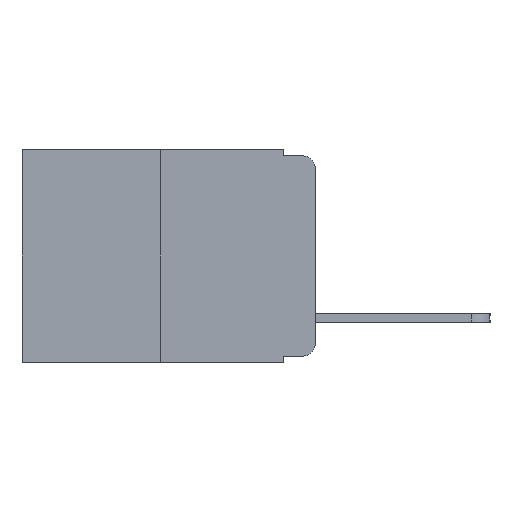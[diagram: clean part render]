
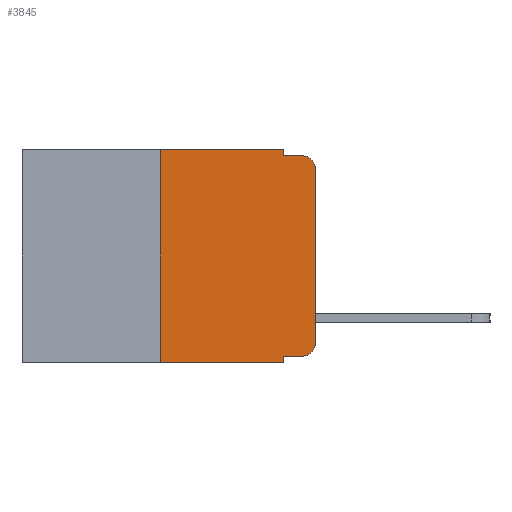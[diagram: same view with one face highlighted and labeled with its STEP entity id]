
A CAD part, left-side view. The second image highlights one B-rep face of the part: STEP entity #3845.
In plain terms, the highlighted planar face has unit normal (-1, 0, 0).
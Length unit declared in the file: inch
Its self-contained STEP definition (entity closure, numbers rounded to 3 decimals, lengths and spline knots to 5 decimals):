
#134 = LINE ( 'NONE', #8582, #2437 ) ;
#140 = DIRECTION ( 'NONE',  ( 0., 0., -1. ) ) ;
#156 = AXIS2_PLACEMENT_3D ( 'NONE', #11019, #10996, #140 ) ;
#361 = ORIENTED_EDGE ( 'NONE', *, *, #5059, .F. ) ;
#370 = EDGE_CURVE ( 'NONE', #8554, #5490, #8906, .T. ) ;
#507 = VECTOR ( 'NONE', #10525, 39.37008 ) ;
#879 = EDGE_CURVE ( 'NONE', #2449, #7760, #5475, .T. ) ;
#1166 = ORIENTED_EDGE ( 'NONE', *, *, #9268, .T. ) ;
#1255 = VERTEX_POINT ( 'NONE', #6982 ) ;
#1303 = CARTESIAN_POINT ( 'NONE',  ( 0., 0.051, -0.333 ) ) ;
#1473 = ORIENTED_EDGE ( 'NONE', *, *, #1939, .T. ) ;
#1610 = EDGE_CURVE ( 'NONE', #2449, #7547, #134, .T. ) ;
#1615 = ORIENTED_EDGE ( 'NONE', *, *, #8835, .F. ) ;
#1650 = CARTESIAN_POINT ( 'NONE',  ( 0., 0., 0. ) ) ;
#1878 = EDGE_CURVE ( 'NONE', #9901, #1255, #3723, .T. ) ;
#1939 = EDGE_CURVE ( 'NONE', #5402, #5490, #5911, .T. ) ;
#1946 = LINE ( 'NONE', #7450, #8960 ) ;
#2437 = VECTOR ( 'NONE', #9664, 39.37008 ) ;
#2449 = VERTEX_POINT ( 'NONE', #6553 ) ;
#2510 = CARTESIAN_POINT ( 'NONE',  ( 0., 0.02, -0.313 ) ) ;
#3001 = AXIS2_PLACEMENT_3D ( 'NONE', #9439, #4034, #8650 ) ;
#3351 = ORIENTED_EDGE ( 'NONE', *, *, #1610, .T. ) ;
#3541 = VECTOR ( 'NONE', #6792, 39.37008 ) ;
#3632 = EDGE_CURVE ( 'NONE', #7420, #9901, #7982, .T. ) ;
#3723 = CIRCLE ( 'NONE', #7213, 0.02 ) ;
#3845 = ADVANCED_FACE ( 'NONE', ( #10465 ), #3967, .F. ) ;
#3888 = DIRECTION ( 'NONE',  ( 0., -1., 0. ) ) ;
#3967 = PLANE ( 'NONE',  #3001 ) ;
#4014 = DIRECTION ( 'NONE',  ( -1., 0., 0. ) ) ;
#4034 = DIRECTION ( 'NONE',  ( 1., 0., 0. ) ) ;
#4139 = VECTOR ( 'NONE', #6726, 39.37008 ) ;
#4362 = CARTESIAN_POINT ( 'NONE',  ( 0., 0.02, -0.333 ) ) ;
#4718 = EDGE_LOOP ( 'NONE', ( #1166, #1473, #6647, #361, #1615, #7304, #3351, #10677, #11140, #6540 ) ) ;
#5059 = EDGE_CURVE ( 'NONE', #5108, #8554, #8701, .T. ) ;
#5108 = VERTEX_POINT ( 'NONE', #5392 ) ;
#5392 = CARTESIAN_POINT ( 'NONE',  ( 0., 0.051, 0. ) ) ;
#5402 = VERTEX_POINT ( 'NONE', #11306 ) ;
#5475 = LINE ( 'NONE', #7705, #7776 ) ;
#5490 = VERTEX_POINT ( 'NONE', #9928 ) ;
#5911 = CIRCLE ( 'NONE', #156, 0.02 ) ;
#6045 = EDGE_CURVE ( 'NONE', #7420, #7547, #7545, .T. ) ;
#6300 = CARTESIAN_POINT ( 'NONE',  ( 0., 0.051, 0. ) ) ;
#6540 = ORIENTED_EDGE ( 'NONE', *, *, #1878, .T. ) ;
#6553 = CARTESIAN_POINT ( 'NONE',  ( 0., 0.25, -0.343 ) ) ;
#6647 = ORIENTED_EDGE ( 'NONE', *, *, #370, .F. ) ;
#6726 = DIRECTION ( 'NONE',  ( 0., 0., -1. ) ) ;
#6792 = DIRECTION ( 'NONE',  ( 0., -1., 0. ) ) ;
#6801 = VECTOR ( 'NONE', #7093, 39.37008 ) ;
#6982 = CARTESIAN_POINT ( 'NONE',  ( 0., 0., -0.313 ) ) ;
#7093 = DIRECTION ( 'NONE',  ( 0., 0., 1. ) ) ;
#7213 = AXIS2_PLACEMENT_3D ( 'NONE', #2510, #4014, #7585 ) ;
#7268 = CARTESIAN_POINT ( 'NONE',  ( 0., 0.25, 0. ) ) ;
#7304 = ORIENTED_EDGE ( 'NONE', *, *, #879, .F. ) ;
#7420 = VERTEX_POINT ( 'NONE', #1303 ) ;
#7430 = CARTESIAN_POINT ( 'NONE',  ( 0., 0.051, -0.01 ) ) ;
#7450 = CARTESIAN_POINT ( 'NONE',  ( 0., 0.473, 0. ) ) ;
#7545 = LINE ( 'NONE', #9716, #507 ) ;
#7547 = VERTEX_POINT ( 'NONE', #8622 ) ;
#7585 = DIRECTION ( 'NONE',  ( 0., 0., -1. ) ) ;
#7705 = CARTESIAN_POINT ( 'NONE',  ( 0., 0.25, 0. ) ) ;
#7760 = VERTEX_POINT ( 'NONE', #7268 ) ;
#7776 = VECTOR ( 'NONE', #9602, 39.37008 ) ;
#7982 = LINE ( 'NONE', #10698, #3541 ) ;
#8554 = VERTEX_POINT ( 'NONE', #10767 ) ;
#8582 = CARTESIAN_POINT ( 'NONE',  ( 0., 0.473, -0.343 ) ) ;
#8622 = CARTESIAN_POINT ( 'NONE',  ( 0., 0.051, -0.343 ) ) ;
#8650 = DIRECTION ( 'NONE',  ( 0., 0., -1. ) ) ;
#8701 = LINE ( 'NONE', #6300, #4139 ) ;
#8835 = EDGE_CURVE ( 'NONE', #7760, #5108, #1946, .T. ) ;
#8906 = LINE ( 'NONE', #7430, #10252 ) ;
#8952 = LINE ( 'NONE', #1650, #6801 ) ;
#8960 = VECTOR ( 'NONE', #3888, 39.37008 ) ;
#9268 = EDGE_CURVE ( 'NONE', #1255, #5402, #8952, .T. ) ;
#9439 = CARTESIAN_POINT ( 'NONE',  ( 0., 0.473, 0. ) ) ;
#9602 = DIRECTION ( 'NONE',  ( 0., 0., 1. ) ) ;
#9664 = DIRECTION ( 'NONE',  ( 0., -1., 0. ) ) ;
#9716 = CARTESIAN_POINT ( 'NONE',  ( 0., 0.051, 0. ) ) ;
#9901 = VERTEX_POINT ( 'NONE', #4362 ) ;
#9928 = CARTESIAN_POINT ( 'NONE',  ( 0., 0.02, -0.01 ) ) ;
#10252 = VECTOR ( 'NONE', #10721, 39.37008 ) ;
#10465 = FACE_OUTER_BOUND ( 'NONE', #4718, .T. ) ;
#10525 = DIRECTION ( 'NONE',  ( 0., 0., -1. ) ) ;
#10677 = ORIENTED_EDGE ( 'NONE', *, *, #6045, .F. ) ;
#10698 = CARTESIAN_POINT ( 'NONE',  ( 0., 0.051, -0.333 ) ) ;
#10721 = DIRECTION ( 'NONE',  ( 0., -1., 0. ) ) ;
#10767 = CARTESIAN_POINT ( 'NONE',  ( 0., 0.051, -0.01 ) ) ;
#10996 = DIRECTION ( 'NONE',  ( -1., 0., 0. ) ) ;
#11019 = CARTESIAN_POINT ( 'NONE',  ( 0., 0.02, -0.03 ) ) ;
#11140 = ORIENTED_EDGE ( 'NONE', *, *, #3632, .T. ) ;
#11306 = CARTESIAN_POINT ( 'NONE',  ( 0., 0., -0.03 ) ) ;
